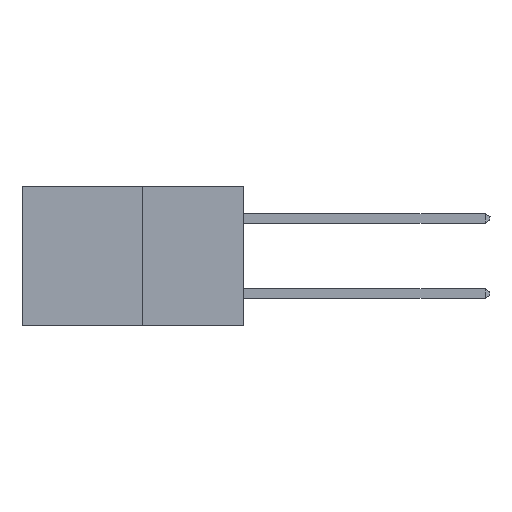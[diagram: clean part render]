
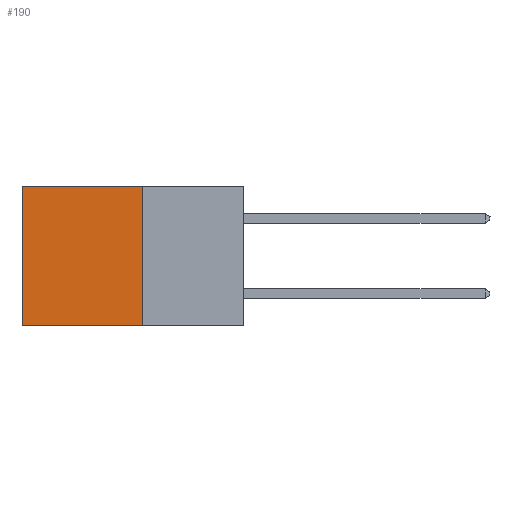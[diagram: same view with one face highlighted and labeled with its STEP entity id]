
A CAD part, left-side view. The second image highlights one B-rep face of the part: STEP entity #190.
In plain terms, the highlighted planar face has unit normal (-1, 0, 0).
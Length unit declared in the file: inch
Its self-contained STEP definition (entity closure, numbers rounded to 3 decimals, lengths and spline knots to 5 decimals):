
#190 = ADVANCED_FACE ( 'NONE', ( #3839 ), #11995, .F. ) ;
#780 = AXIS2_PLACEMENT_3D ( 'NONE', #4910, #7917, #8448 ) ;
#823 = CARTESIAN_POINT ( 'NONE',  ( 0.277, 0.27, 0. ) ) ;
#1150 = ORIENTED_EDGE ( 'NONE', *, *, #6688, .F. ) ;
#1456 = VECTOR ( 'NONE', #6815, 39.37008 ) ;
#1675 = VERTEX_POINT ( 'NONE', #3100 ) ;
#1816 = LINE ( 'NONE', #9118, #1456 ) ;
#3100 = CARTESIAN_POINT ( 'NONE',  ( 0.277, 0.59, -0.37 ) ) ;
#3731 = VECTOR ( 'NONE', #5242, 39.37008 ) ;
#3839 = FACE_OUTER_BOUND ( 'NONE', #8456, .T. ) ;
#3891 = ORIENTED_EDGE ( 'NONE', *, *, #9166, .T. ) ;
#4910 = CARTESIAN_POINT ( 'NONE',  ( 0.277, 0.27, -0.37 ) ) ;
#4968 = ORIENTED_EDGE ( 'NONE', *, *, #6012, .F. ) ;
#5136 = VERTEX_POINT ( 'NONE', #823 ) ;
#5147 = CARTESIAN_POINT ( 'NONE',  ( 0.277, 0.59, -0.37 ) ) ;
#5242 = DIRECTION ( 'NONE',  ( 0., 0., -1. ) ) ;
#5309 = VERTEX_POINT ( 'NONE', #10551 ) ;
#6012 = EDGE_CURVE ( 'NONE', #5136, #5309, #1816, .T. ) ;
#6688 = EDGE_CURVE ( 'NONE', #5309, #1675, #13243, .T. ) ;
#6815 = DIRECTION ( 'NONE',  ( 0., 0., -1. ) ) ;
#6964 = VECTOR ( 'NONE', #8071, 39.37008 ) ;
#7566 = VERTEX_POINT ( 'NONE', #9115 ) ;
#7674 = CARTESIAN_POINT ( 'NONE',  ( 0.277, 0.27, -0.37 ) ) ;
#7917 = DIRECTION ( 'NONE',  ( 1., 0., 0. ) ) ;
#7995 = ORIENTED_EDGE ( 'NONE', *, *, #8520, .T. ) ;
#8071 = DIRECTION ( 'NONE',  ( 0., 1., 0. ) ) ;
#8151 = CARTESIAN_POINT ( 'NONE',  ( 0.277, 0.27, 0. ) ) ;
#8448 = DIRECTION ( 'NONE',  ( 0., 0., -1. ) ) ;
#8456 = EDGE_LOOP ( 'NONE', ( #3891, #1150, #4968, #7995 ) ) ;
#8520 = EDGE_CURVE ( 'NONE', #5136, #7566, #9958, .T. ) ;
#9115 = CARTESIAN_POINT ( 'NONE',  ( 0.277, 0.59, 0. ) ) ;
#9118 = CARTESIAN_POINT ( 'NONE',  ( 0.277, 0.27, -0.37 ) ) ;
#9166 = EDGE_CURVE ( 'NONE', #7566, #1675, #12697, .T. ) ;
#9958 = LINE ( 'NONE', #8151, #6964 ) ;
#10367 = VECTOR ( 'NONE', #12444, 39.37008 ) ;
#10551 = CARTESIAN_POINT ( 'NONE',  ( 0.277, 0.27, -0.37 ) ) ;
#11995 = PLANE ( 'NONE',  #780 ) ;
#12444 = DIRECTION ( 'NONE',  ( 0., 1., 0. ) ) ;
#12697 = LINE ( 'NONE', #5147, #3731 ) ;
#13243 = LINE ( 'NONE', #7674, #10367 ) ;
